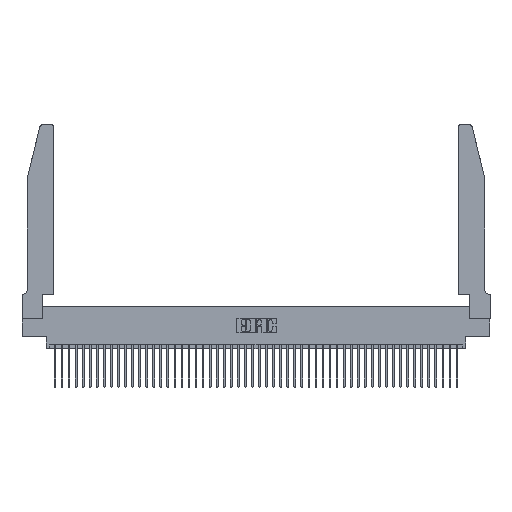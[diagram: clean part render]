
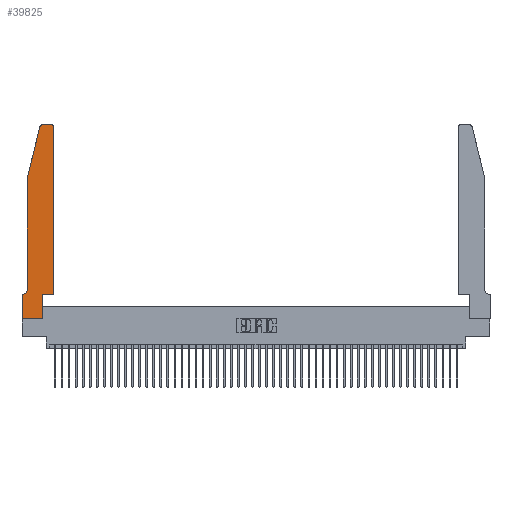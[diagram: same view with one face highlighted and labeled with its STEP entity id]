
A CAD part, top view. The second image highlights one B-rep face of the part: STEP entity #39825.
In plain terms, the highlighted planar face has unit normal (0, 0, 1).
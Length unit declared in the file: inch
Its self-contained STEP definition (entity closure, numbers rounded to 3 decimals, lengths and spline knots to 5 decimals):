
#616 = CARTESIAN_POINT ( 'NONE',  ( 0.2865, 0.35, 0.37 ) ) ;
#942 = CARTESIAN_POINT ( 'NONE',  ( 0.284, 2.72, 0.37 ) ) ;
#974 = DIRECTION ( 'NONE',  ( 1., 0., 0. ) ) ;
#989 = CIRCLE ( 'NONE', #16788, 0.03 ) ;
#1134 = DIRECTION ( 'NONE',  ( -1., 0., 0. ) ) ;
#1332 = LINE ( 'NONE', #47215, #30090 ) ;
#1908 = ORIENTED_EDGE ( 'NONE', *, *, #16708, .T. ) ;
#2145 = CARTESIAN_POINT ( 'NONE',  ( 0., 0.35, 0.37 ) ) ;
#2305 = LINE ( 'NONE', #45716, #40868 ) ;
#3074 = CARTESIAN_POINT ( 'NONE',  ( 0.4505, 2.72, 0.37 ) ) ;
#3293 = EDGE_CURVE ( 'NONE', #23717, #38478, #37031, .T. ) ;
#3808 = DIRECTION ( 'NONE',  ( 0., 0., 1. ) ) ;
#4557 = PLANE ( 'NONE',  #47862 ) ;
#4698 = DIRECTION ( 'NONE',  ( -1., 0., 0. ) ) ;
#4736 = DIRECTION ( 'NONE',  ( 1., 0., 0. ) ) ;
#6602 = CARTESIAN_POINT ( 'NONE',  ( 0.2865, 0., 0.37 ) ) ;
#6687 = ORIENTED_EDGE ( 'NONE', *, *, #45755, .T. ) ;
#6707 = EDGE_CURVE ( 'NONE', #39305, #21201, #989, .T. ) ;
#6816 = VERTEX_POINT ( 'NONE', #30350 ) ;
#6951 = ORIENTED_EDGE ( 'NONE', *, *, #27037, .T. ) ;
#7496 = EDGE_CURVE ( 'NONE', #47325, #19722, #36616, .T. ) ;
#7602 = CIRCLE ( 'NONE', #17670, 0.07 ) ;
#8189 = DIRECTION ( 'NONE',  ( 0., 1., 0. ) ) ;
#8356 = DIRECTION ( 'NONE',  ( 0., 0., 1. ) ) ;
#9334 = CARTESIAN_POINT ( 'NONE',  ( 0., 0., 0.37 ) ) ;
#9368 = EDGE_CURVE ( 'NONE', #36817, #6816, #38241, .T. ) ;
#9566 = VERTEX_POINT ( 'NONE', #14986 ) ;
#9592 = VECTOR ( 'NONE', #4698, 39.37008 ) ;
#9931 = EDGE_LOOP ( 'NONE', ( #46055, #43257, #17550, #36544, #6951, #17211, #24482, #42393, #29889, #6687, #1908, #26026 ) ) ;
#11181 = VECTOR ( 'NONE', #40993, 39.37008 ) ;
#11877 = CARTESIAN_POINT ( 'NONE',  ( 0.0755, 2., 0.37 ) ) ;
#14986 = CARTESIAN_POINT ( 'NONE',  ( 0.4505, 0.35, 0.37 ) ) ;
#16408 = VECTOR ( 'NONE', #974, 39.37008 ) ;
#16708 = EDGE_CURVE ( 'NONE', #9566, #39305, #46371, .T. ) ;
#16788 = AXIS2_PLACEMENT_3D ( 'NONE', #26292, #3808, #30041 ) ;
#17211 = ORIENTED_EDGE ( 'NONE', *, *, #3293, .T. ) ;
#17550 = ORIENTED_EDGE ( 'NONE', *, *, #44684, .T. ) ;
#17670 = AXIS2_PLACEMENT_3D ( 'NONE', #45812, #23667, #1134 ) ;
#19335 = LINE ( 'NONE', #9334, #39017 ) ;
#19722 = VERTEX_POINT ( 'NONE', #47317 ) ;
#20915 = EDGE_CURVE ( 'NONE', #38478, #34769, #19335, .T. ) ;
#21201 = VERTEX_POINT ( 'NONE', #44320 ) ;
#21560 = CARTESIAN_POINT ( 'NONE',  ( 0.4505, 0.35, 0.37 ) ) ;
#21740 = FACE_OUTER_BOUND ( 'NONE', #9931, .T. ) ;
#22189 = CARTESIAN_POINT ( 'NONE',  ( 0.0755, 0.42, 0.37 ) ) ;
#23667 = DIRECTION ( 'NONE',  ( 0., 0., -1. ) ) ;
#23717 = VERTEX_POINT ( 'NONE', #45019 ) ;
#24482 = ORIENTED_EDGE ( 'NONE', *, *, #20915, .T. ) ;
#25582 = VERTEX_POINT ( 'NONE', #22189 ) ;
#26026 = ORIENTED_EDGE ( 'NONE', *, *, #6707, .T. ) ;
#26292 = CARTESIAN_POINT ( 'NONE',  ( 0.4205, 2.72, 0.37 ) ) ;
#26295 = CARTESIAN_POINT ( 'NONE',  ( 0.0755, 0.35, 0.37 ) ) ;
#26940 = EDGE_CURVE ( 'NONE', #45317, #25582, #40880, .T. ) ;
#27037 = EDGE_CURVE ( 'NONE', #25582, #23717, #7602, .T. ) ;
#27181 = CARTESIAN_POINT ( 'NONE',  ( 0.2605, 2.75, 0.37 ) ) ;
#27210 = DIRECTION ( 'NONE',  ( 0., 0., 1. ) ) ;
#27284 = DIRECTION ( 'NONE',  ( 0., 1., 0. ) ) ;
#28356 = VECTOR ( 'NONE', #30043, 39.37008 ) ;
#29889 = ORIENTED_EDGE ( 'NONE', *, *, #7496, .T. ) ;
#30041 = DIRECTION ( 'NONE',  ( 1., 0., 0. ) ) ;
#30043 = DIRECTION ( 'NONE',  ( -1., 0., 0. ) ) ;
#30090 = VECTOR ( 'NONE', #39813, 39.37008 ) ;
#30324 = CARTESIAN_POINT ( 'NONE',  ( 0.284, 2.75, 0.37 ) ) ;
#30350 = CARTESIAN_POINT ( 'NONE',  ( 0.25487, 2.72718, 0.37 ) ) ;
#30780 = CARTESIAN_POINT ( 'NONE',  ( 0., 0.35, 0.37 ) ) ;
#31024 = DIRECTION ( 'NONE',  ( -0.239, -0.971, 0. ) ) ;
#33570 = EDGE_CURVE ( 'NONE', #34769, #47325, #1332, .T. ) ;
#34475 = DIRECTION ( 'NONE',  ( 1., 0., 0. ) ) ;
#34769 = VERTEX_POINT ( 'NONE', #47424 ) ;
#35443 = DIRECTION ( 'NONE',  ( 0., -1., 0. ) ) ;
#36544 = ORIENTED_EDGE ( 'NONE', *, *, #26940, .T. ) ;
#36616 = LINE ( 'NONE', #616, #45268 ) ;
#36817 = VERTEX_POINT ( 'NONE', #30324 ) ;
#37031 = LINE ( 'NONE', #26295, #28356 ) ;
#37279 = CARTESIAN_POINT ( 'NONE',  ( 0.0755, 2., 0.37 ) ) ;
#37566 = EDGE_CURVE ( 'NONE', #21201, #36817, #38178, .T. ) ;
#38178 = LINE ( 'NONE', #27181, #9592 ) ;
#38241 = CIRCLE ( 'NONE', #40794, 0.03 ) ;
#38272 = CARTESIAN_POINT ( 'NONE',  ( 0.4505, 0.35, 0.37 ) ) ;
#38478 = VERTEX_POINT ( 'NONE', #2145 ) ;
#39017 = VECTOR ( 'NONE', #35443, 39.37008 ) ;
#39305 = VERTEX_POINT ( 'NONE', #3074 ) ;
#39813 = DIRECTION ( 'NONE',  ( 1., 0., 0. ) ) ;
#39825 = ADVANCED_FACE ( 'NONE', ( #21740 ), #4557, .T. ) ;
#40794 = AXIS2_PLACEMENT_3D ( 'NONE', #942, #27210, #4736 ) ;
#40868 = VECTOR ( 'NONE', #31024, 39.37008 ) ;
#40880 = LINE ( 'NONE', #37279, #11181 ) ;
#40993 = DIRECTION ( 'NONE',  ( 0., -1., 0. ) ) ;
#42393 = ORIENTED_EDGE ( 'NONE', *, *, #33570, .T. ) ;
#43257 = ORIENTED_EDGE ( 'NONE', *, *, #9368, .T. ) ;
#44320 = CARTESIAN_POINT ( 'NONE',  ( 0.4205, 2.75, 0.37 ) ) ;
#44684 = EDGE_CURVE ( 'NONE', #6816, #45317, #2305, .T. ) ;
#45019 = CARTESIAN_POINT ( 'NONE',  ( 0.0055, 0.35, 0.37 ) ) ;
#45216 = VECTOR ( 'NONE', #27284, 39.37008 ) ;
#45268 = VECTOR ( 'NONE', #8189, 39.37008 ) ;
#45317 = VERTEX_POINT ( 'NONE', #11877 ) ;
#45716 = CARTESIAN_POINT ( 'NONE',  ( 0.0755, 2., 0.37 ) ) ;
#45755 = EDGE_CURVE ( 'NONE', #19722, #9566, #48249, .T. ) ;
#45812 = CARTESIAN_POINT ( 'NONE',  ( 0.0055, 0.42, 0.37 ) ) ;
#46055 = ORIENTED_EDGE ( 'NONE', *, *, #37566, .T. ) ;
#46371 = LINE ( 'NONE', #38272, #45216 ) ;
#47215 = CARTESIAN_POINT ( 'NONE',  ( 0., 0., 0.37 ) ) ;
#47317 = CARTESIAN_POINT ( 'NONE',  ( 0.2865, 0.35, 0.37 ) ) ;
#47325 = VERTEX_POINT ( 'NONE', #6602 ) ;
#47424 = CARTESIAN_POINT ( 'NONE',  ( 0., 0., 0.37 ) ) ;
#47862 = AXIS2_PLACEMENT_3D ( 'NONE', #30780, #8356, #34475 ) ;
#48249 = LINE ( 'NONE', #21560, #16408 ) ;
